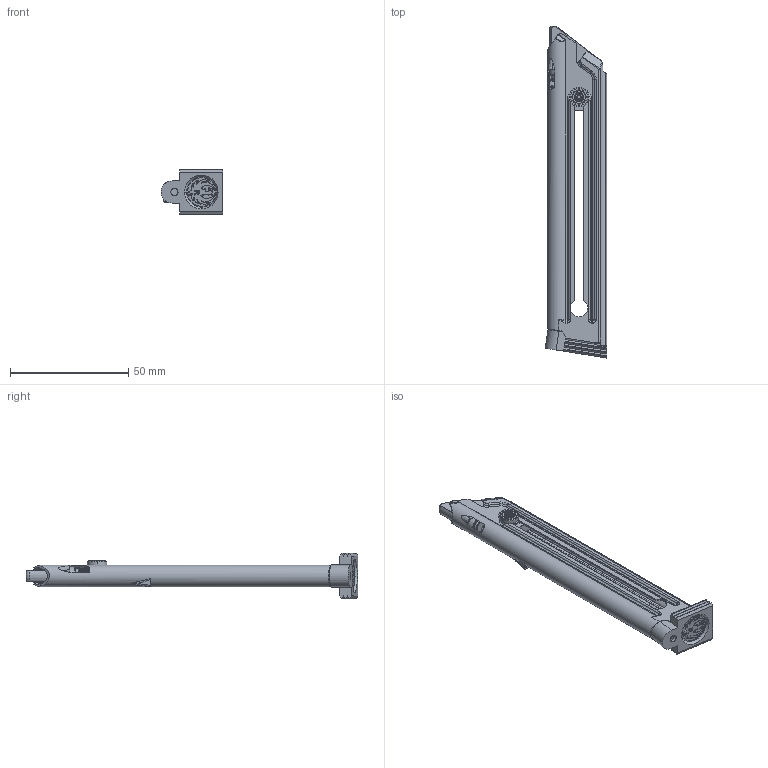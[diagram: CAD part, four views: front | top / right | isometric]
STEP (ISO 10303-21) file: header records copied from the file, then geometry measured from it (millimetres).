
FILE_DESCRIPTION((''),'2;1');
FILE_NAME('MAGAZINE_ASM','2011-09-26T',('how300060'),(''),'PRO/ENGINEER BY PARAMETRIC TECHNOLOGY CORPORATION, 2011040','PRO/ENGINEER BY PARAMETRIC TECHNOLOGY CORPORATION, 2011040','');
FILE_SCHEMA(('CONFIG_CONTROL_DESIGN'));
Length unit declared in the file: inch
Products named in the file (7): MAGAZINE-BODY; MAGAZINE-FOLLOWER; MAGAZINE-FOLLOWER-BUTTON; MAGAZINE-BASE-PLATE; MAGAZINE-SPRING-PLUNGER; MAGAZINE-SPRING_AF0; MAGAZINE_ASM
Assembly tree (6 placements, depth 2):
  MAGAZINE_ASM
    MAGAZINE-BODY
    MAGAZINE-FOLLOWER
    MAGAZINE-FOLLOWER-BUTTON
    MAGAZINE-BASE-PLATE
    MAGAZINE-SPRING-PLUNGER
    MAGAZINE-SPRING_AF0
Bounding box: 26.09 x 140.13 x 19.13 mm (x, y, z)
Volume: 10005.6 mm3; surface area: 19445.4 mm2
Topology: 6 solids, 6 shells, 602 faces, 1528 edges, 953 vertices
Faces by surface type: cylinder 206, plane 194, torus 66, bspline 62, extrusion 40, sphere 20, cone 14
Entity records: 38728 total; most frequent: CARTESIAN_POINT 19595, ORIENTED_EDGE 3056, DIRECTION 2743, PRESENTATION_STYLE_ASSIGNMENT 1542, STYLED_ITEM 1534, CURVE_STYLE 1528, EDGE_CURVE 1528, AXIS2_PLACEMENT_3D 999
